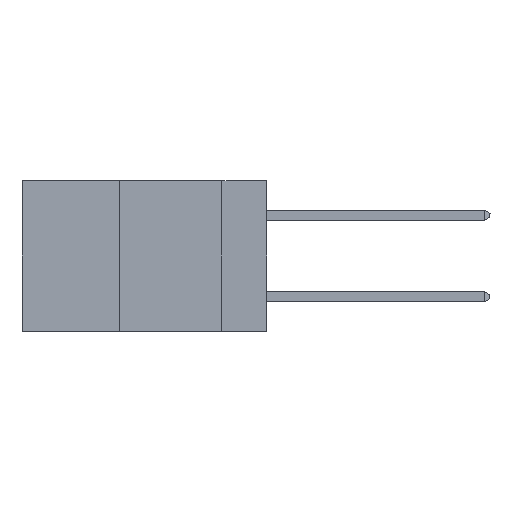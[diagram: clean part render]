
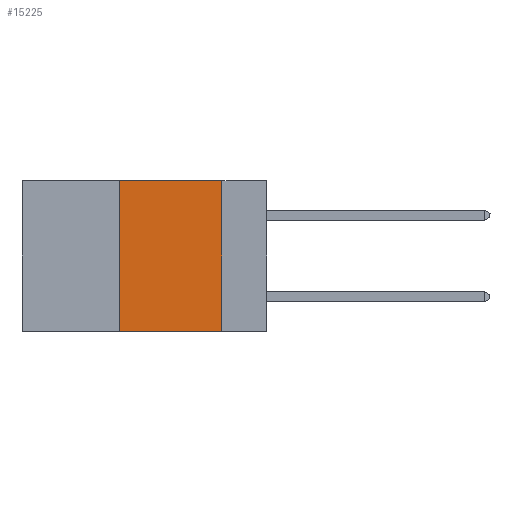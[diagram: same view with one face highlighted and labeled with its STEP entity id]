
A CAD part, left-side view. The second image highlights one B-rep face of the part: STEP entity #15225.
In plain terms, the highlighted planar face has unit normal (-1, 0, 0).
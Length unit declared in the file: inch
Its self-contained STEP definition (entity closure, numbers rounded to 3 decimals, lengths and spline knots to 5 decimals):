
#1517 = LINE ( 'NONE', #35011, #27163 ) ;
#2995 = DIRECTION ( 'NONE',  ( 0., 0., -1. ) ) ;
#6692 = DIRECTION ( 'NONE',  ( 0., 0., 1. ) ) ;
#9374 = VERTEX_POINT ( 'NONE', #37746 ) ;
#9833 = CARTESIAN_POINT ( 'NONE',  ( 0., 0.11, 0. ) ) ;
#10110 = ORIENTED_EDGE ( 'NONE', *, *, #22114, .F. ) ;
#11531 = DIRECTION ( 'NONE',  ( 0., -1., 0. ) ) ;
#12246 = EDGE_CURVE ( 'NONE', #32870, #9374, #1517, .T. ) ;
#14147 = CARTESIAN_POINT ( 'NONE',  ( 0., 0.6, 0. ) ) ;
#15225 = ADVANCED_FACE ( 'NONE', ( #41170 ), #19504, .F. ) ;
#15688 = LINE ( 'NONE', #14147, #23560 ) ;
#16447 = CARTESIAN_POINT ( 'NONE',  ( 0., 0.36, 0. ) ) ;
#16535 = AXIS2_PLACEMENT_3D ( 'NONE', #43163, #23040, #2995 ) ;
#17232 = ORIENTED_EDGE ( 'NONE', *, *, #37007, .F. ) ;
#18006 = EDGE_LOOP ( 'NONE', ( #10110, #34764, #17232, #18748 ) ) ;
#18748 = ORIENTED_EDGE ( 'NONE', *, *, #12246, .T. ) ;
#19504 = PLANE ( 'NONE',  #16535 ) ;
#20132 = CARTESIAN_POINT ( 'NONE',  ( 0., 0.36, 0. ) ) ;
#20234 = CARTESIAN_POINT ( 'NONE',  ( 0., 0.11, 0. ) ) ;
#20687 = VERTEX_POINT ( 'NONE', #9833 ) ;
#21587 = CARTESIAN_POINT ( 'NONE',  ( 0., 0.36, -0.37 ) ) ;
#22114 = EDGE_CURVE ( 'NONE', #20687, #9374, #43005, .T. ) ;
#23040 = DIRECTION ( 'NONE',  ( 1., 0., 0. ) ) ;
#23560 = VECTOR ( 'NONE', #34257, 39.37008 ) ;
#25143 = VECTOR ( 'NONE', #37039, 39.37008 ) ;
#26153 = VERTEX_POINT ( 'NONE', #16447 ) ;
#27163 = VECTOR ( 'NONE', #11531, 39.37008 ) ;
#29914 = LINE ( 'NONE', #20132, #37807 ) ;
#32870 = VERTEX_POINT ( 'NONE', #21587 ) ;
#34257 = DIRECTION ( 'NONE',  ( 0., -1., 0. ) ) ;
#34764 = ORIENTED_EDGE ( 'NONE', *, *, #37151, .F. ) ;
#35011 = CARTESIAN_POINT ( 'NONE',  ( 0., 0.6, -0.37 ) ) ;
#37007 = EDGE_CURVE ( 'NONE', #32870, #26153, #29914, .T. ) ;
#37039 = DIRECTION ( 'NONE',  ( 0., 0., -1. ) ) ;
#37151 = EDGE_CURVE ( 'NONE', #26153, #20687, #15688, .T. ) ;
#37746 = CARTESIAN_POINT ( 'NONE',  ( 0., 0.11, -0.37 ) ) ;
#37807 = VECTOR ( 'NONE', #6692, 39.37008 ) ;
#41170 = FACE_OUTER_BOUND ( 'NONE', #18006, .T. ) ;
#43005 = LINE ( 'NONE', #20234, #25143 ) ;
#43163 = CARTESIAN_POINT ( 'NONE',  ( 0., 0.6, 0. ) ) ;
